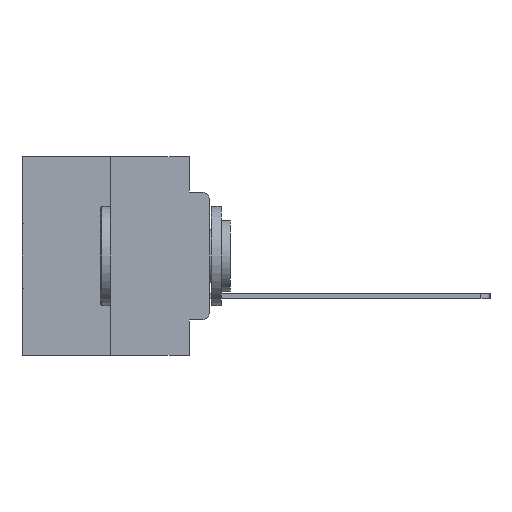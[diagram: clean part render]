
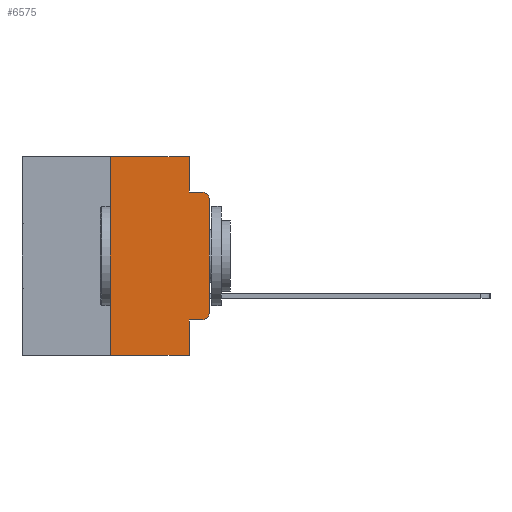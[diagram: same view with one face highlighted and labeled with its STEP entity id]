
A CAD part, left-side view. The second image highlights one B-rep face of the part: STEP entity #6575.
In plain terms, the highlighted planar face has unit normal (-1, 0, 0).
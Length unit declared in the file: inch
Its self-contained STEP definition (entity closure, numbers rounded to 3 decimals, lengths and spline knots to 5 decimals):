
#179 = VERTEX_POINT ( 'NONE', #26442 ) ;
#452 = VECTOR ( 'NONE', #21825, 39.37008 ) ;
#1257 = VERTEX_POINT ( 'NONE', #26964 ) ;
#1631 = CARTESIAN_POINT ( 'NONE',  ( 0., 0.25, 0. ) ) ;
#2441 = VERTEX_POINT ( 'NONE', #4169 ) ;
#3600 = CARTESIAN_POINT ( 'NONE',  ( 0., 0., -0.1085 ) ) ;
#3823 = EDGE_CURVE ( 'NONE', #4751, #10393, #20265, .T. ) ;
#3902 = ORIENTED_EDGE ( 'NONE', *, *, #5541, .T. ) ;
#4169 = CARTESIAN_POINT ( 'NONE',  ( 0., 0.051, 0. ) ) ;
#4409 = CARTESIAN_POINT ( 'NONE',  ( 0., 0.02, -0.1085 ) ) ;
#4485 = VERTEX_POINT ( 'NONE', #19363 ) ;
#4751 = VERTEX_POINT ( 'NONE', #13064 ) ;
#5541 = EDGE_CURVE ( 'NONE', #1257, #4751, #29747, .T. ) ;
#6243 = CARTESIAN_POINT ( 'NONE',  ( 0., 0.473, 0. ) ) ;
#6575 = ADVANCED_FACE ( 'NONE', ( #27464 ), #23436, .F. ) ;
#6578 = EDGE_CURVE ( 'NONE', #29175, #10794, #21219, .T. ) ;
#6694 = EDGE_LOOP ( 'NONE', ( #28858, #15276, #12727, #21169, #24139, #16451, #11645, #13128, #3902, #18001 ) ) ;
#6942 = DIRECTION ( 'NONE',  ( 0., 0., -1. ) ) ;
#8812 = DIRECTION ( 'NONE',  ( 0., 0., -1. ) ) ;
#9345 = CARTESIAN_POINT ( 'NONE',  ( 0., 0.473, 0. ) ) ;
#9436 = DIRECTION ( 'NONE',  ( -1., 0., 0. ) ) ;
#9844 = CARTESIAN_POINT ( 'NONE',  ( 0., 0.051, -0.4115 ) ) ;
#9951 = DIRECTION ( 'NONE',  ( 0., -1., 0. ) ) ;
#9999 = CARTESIAN_POINT ( 'NONE',  ( 0., 0.051, -0.0885 ) ) ;
#10108 = CARTESIAN_POINT ( 'NONE',  ( 0., 0.473, -0.5 ) ) ;
#10393 = VERTEX_POINT ( 'NONE', #16724 ) ;
#10794 = VERTEX_POINT ( 'NONE', #30008 ) ;
#11099 = DIRECTION ( 'NONE',  ( 0., -1., 0. ) ) ;
#11268 = CARTESIAN_POINT ( 'NONE',  ( 0., 0.051, 0. ) ) ;
#11428 = VECTOR ( 'NONE', #8812, 39.37008 ) ;
#11518 = EDGE_CURVE ( 'NONE', #10393, #29175, #26634, .T. ) ;
#11645 = ORIENTED_EDGE ( 'NONE', *, *, #20616, .T. ) ;
#11749 = DIRECTION ( 'NONE',  ( 1., 0., 0. ) ) ;
#12030 = DIRECTION ( 'NONE',  ( 0., 0., -1. ) ) ;
#12398 = DIRECTION ( 'NONE',  ( 0., -1., 0. ) ) ;
#12691 = DIRECTION ( 'NONE',  ( 0., 0., 1. ) ) ;
#12727 = ORIENTED_EDGE ( 'NONE', *, *, #30975, .F. ) ;
#13064 = CARTESIAN_POINT ( 'NONE',  ( 0., 0.02, -0.4115 ) ) ;
#13128 = ORIENTED_EDGE ( 'NONE', *, *, #13674, .F. ) ;
#13376 = CARTESIAN_POINT ( 'NONE',  ( 0., 0.25, -0.5 ) ) ;
#13384 = VECTOR ( 'NONE', #12691, 39.37008 ) ;
#13674 = EDGE_CURVE ( 'NONE', #1257, #179, #30173, .T. ) ;
#14473 = VECTOR ( 'NONE', #12030, 39.37008 ) ;
#15058 = CARTESIAN_POINT ( 'NONE',  ( 0., 0., 0. ) ) ;
#15276 = ORIENTED_EDGE ( 'NONE', *, *, #6578, .T. ) ;
#15281 = EDGE_CURVE ( 'NONE', #25919, #4485, #20171, .T. ) ;
#16322 = DIRECTION ( 'NONE',  ( 0., 0., 1. ) ) ;
#16451 = ORIENTED_EDGE ( 'NONE', *, *, #15281, .F. ) ;
#16724 = CARTESIAN_POINT ( 'NONE',  ( 0., 0., -0.3915 ) ) ;
#17295 = VECTOR ( 'NONE', #9951, 39.37008 ) ;
#17742 = AXIS2_PLACEMENT_3D ( 'NONE', #23543, #9436, #25946 ) ;
#17762 = LINE ( 'NONE', #9999, #29492 ) ;
#18001 = ORIENTED_EDGE ( 'NONE', *, *, #3823, .T. ) ;
#18379 = LINE ( 'NONE', #6243, #30822 ) ;
#19041 = CARTESIAN_POINT ( 'NONE',  ( 0., 0.051, -0.0885 ) ) ;
#19363 = CARTESIAN_POINT ( 'NONE',  ( 0., 0.25, 0. ) ) ;
#19915 = LINE ( 'NONE', #10108, #452 ) ;
#20171 = LINE ( 'NONE', #1631, #26405 ) ;
#20265 = CIRCLE ( 'NONE', #17742, 0.02 ) ;
#20616 = EDGE_CURVE ( 'NONE', #25919, #179, #19915, .T. ) ;
#21169 = ORIENTED_EDGE ( 'NONE', *, *, #24699, .F. ) ;
#21214 = DIRECTION ( 'NONE',  ( -1., 0., 0. ) ) ;
#21219 = CIRCLE ( 'NONE', #28168, 0.02 ) ;
#21825 = DIRECTION ( 'NONE',  ( 0., -1., 0. ) ) ;
#22028 = VERTEX_POINT ( 'NONE', #19041 ) ;
#23436 = PLANE ( 'NONE',  #29750 ) ;
#23543 = CARTESIAN_POINT ( 'NONE',  ( 0., 0.02, -0.3915 ) ) ;
#24139 = ORIENTED_EDGE ( 'NONE', *, *, #26959, .F. ) ;
#24699 = EDGE_CURVE ( 'NONE', #2441, #22028, #26965, .T. ) ;
#25919 = VERTEX_POINT ( 'NONE', #13376 ) ;
#25946 = DIRECTION ( 'NONE',  ( 0., 0., -1. ) ) ;
#26103 = CARTESIAN_POINT ( 'NONE',  ( 0., 0.051, 0. ) ) ;
#26405 = VECTOR ( 'NONE', #16322, 39.37008 ) ;
#26442 = CARTESIAN_POINT ( 'NONE',  ( 0., 0.051, -0.5 ) ) ;
#26634 = LINE ( 'NONE', #15058, #13384 ) ;
#26959 = EDGE_CURVE ( 'NONE', #4485, #2441, #18379, .T. ) ;
#26964 = CARTESIAN_POINT ( 'NONE',  ( 0., 0.051, -0.4115 ) ) ;
#26965 = LINE ( 'NONE', #26103, #14473 ) ;
#27464 = FACE_OUTER_BOUND ( 'NONE', #6694, .T. ) ;
#28168 = AXIS2_PLACEMENT_3D ( 'NONE', #4409, #21214, #6942 ) ;
#28208 = DIRECTION ( 'NONE',  ( 0., 0., -1. ) ) ;
#28858 = ORIENTED_EDGE ( 'NONE', *, *, #11518, .T. ) ;
#29175 = VERTEX_POINT ( 'NONE', #3600 ) ;
#29492 = VECTOR ( 'NONE', #12398, 39.37008 ) ;
#29747 = LINE ( 'NONE', #9844, #17295 ) ;
#29750 = AXIS2_PLACEMENT_3D ( 'NONE', #9345, #11749, #28208 ) ;
#30008 = CARTESIAN_POINT ( 'NONE',  ( 0., 0.02, -0.0885 ) ) ;
#30173 = LINE ( 'NONE', #11268, #11428 ) ;
#30822 = VECTOR ( 'NONE', #11099, 39.37008 ) ;
#30975 = EDGE_CURVE ( 'NONE', #22028, #10794, #17762, .T. ) ;
